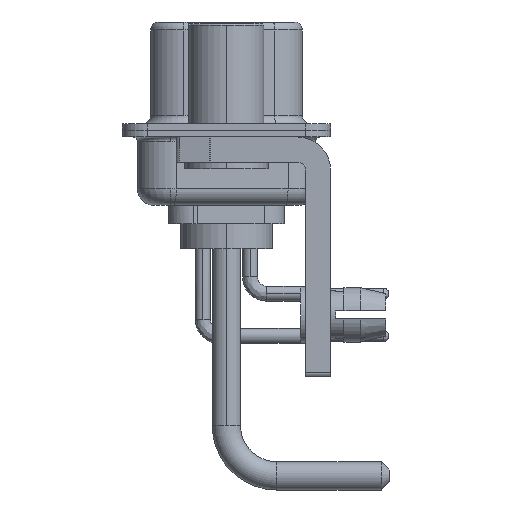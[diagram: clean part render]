
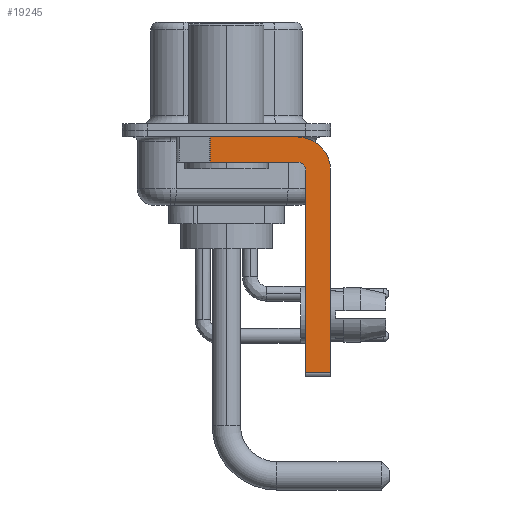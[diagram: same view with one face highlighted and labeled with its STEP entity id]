
A CAD part, left-side view. The second image highlights one B-rep face of the part: STEP entity #19245.
In plain terms, the highlighted planar face has unit normal (-1, 0, 0).
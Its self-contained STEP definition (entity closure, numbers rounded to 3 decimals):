
#707 = EDGE_CURVE ( 'NONE', #15622, #6679, #5319, .T. ) ;
#946 = CARTESIAN_POINT ( 'NONE',  ( -2.9, -4.75, -14.8 ) ) ;
#1296 = EDGE_CURVE ( 'NONE', #25440, #26084, #15263, .T. ) ;
#2064 = LINE ( 'NONE', #4436, #20215 ) ;
#2780 = VERTEX_POINT ( 'NONE', #26372 ) ;
#3285 = PLANE ( 'NONE',  #5467 ) ;
#3473 = DIRECTION ( 'NONE',  ( 0., 0., -1. ) ) ;
#4436 = CARTESIAN_POINT ( 'NONE',  ( -2.9, 3., -0.4 ) ) ;
#4575 = DIRECTION ( 'NONE',  ( 0., -1., 0. ) ) ;
#4729 = EDGE_CURVE ( 'NONE', #21478, #20223, #9816, .T. ) ;
#5319 = LINE ( 'NONE', #7099, #14915 ) ;
#5467 = AXIS2_PLACEMENT_3D ( 'NONE', #16999, #21433, #21286 ) ;
#5736 = ORIENTED_EDGE ( 'NONE', *, *, #15681, .F. ) ;
#5931 = DIRECTION ( 'NONE',  ( 0., 1., 0. ) ) ;
#6679 = VERTEX_POINT ( 'NONE', #17961 ) ;
#7099 = CARTESIAN_POINT ( 'NONE',  ( -2.9, 0.978, -1.9 ) ) ;
#7449 = DIRECTION ( 'NONE',  ( 0., 0., 1. ) ) ;
#7663 = CARTESIAN_POINT ( 'NONE',  ( -2.9, -4.25, -2.4 ) ) ;
#8130 = LINE ( 'NONE', #10212, #20425 ) ;
#9448 = DIRECTION ( 'NONE',  ( -1., 0., 0. ) ) ;
#9508 = CARTESIAN_POINT ( 'NONE',  ( -2.9, -4.25, -2.4 ) ) ;
#9785 = VECTOR ( 'NONE', #3473, 1000. ) ;
#9816 = LINE ( 'NONE', #946, #11301 ) ;
#9962 = VECTOR ( 'NONE', #14003, 1000. ) ;
#10212 = CARTESIAN_POINT ( 'NONE',  ( -2.9, -4.25, -1.9 ) ) ;
#11301 = VECTOR ( 'NONE', #7449, 1000. ) ;
#11596 = CARTESIAN_POINT ( 'NONE',  ( -2.9, -6.25, -2.4 ) ) ;
#11713 = EDGE_CURVE ( 'NONE', #21478, #26084, #15914, .T. ) ;
#12149 = FACE_OUTER_BOUND ( 'NONE', #17409, .T. ) ;
#13572 = CARTESIAN_POINT ( 'NONE',  ( -2.9, -4.25, -14.55 ) ) ;
#13869 = DIRECTION ( 'NONE',  ( 0., 0., 1. ) ) ;
#13924 = DIRECTION ( 'NONE',  ( 1., 0., 0. ) ) ;
#14003 = DIRECTION ( 'NONE',  ( 0., -1., 0. ) ) ;
#14226 = EDGE_CURVE ( 'NONE', #15622, #17719, #2064, .T. ) ;
#14915 = VECTOR ( 'NONE', #25531, 1000. ) ;
#15263 = LINE ( 'NONE', #21460, #9785 ) ;
#15462 = EDGE_CURVE ( 'NONE', #2780, #6679, #8130, .T. ) ;
#15622 = VERTEX_POINT ( 'NONE', #15921 ) ;
#15681 = EDGE_CURVE ( 'NONE', #20223, #2780, #28939, .T. ) ;
#15913 = ORIENTED_EDGE ( 'NONE', *, *, #14226, .F. ) ;
#15914 = LINE ( 'NONE', #13572, #9962 ) ;
#15921 = CARTESIAN_POINT ( 'NONE',  ( -2.9, 0.978, -0.4 ) ) ;
#16760 = ORIENTED_EDGE ( 'NONE', *, *, #11713, .T. ) ;
#16999 = CARTESIAN_POINT ( 'NONE',  ( -2.9, -4.25, -2.4 ) ) ;
#17387 = CARTESIAN_POINT ( 'NONE',  ( -2.9, -6.25, -14.55 ) ) ;
#17409 = EDGE_LOOP ( 'NONE', ( #15913, #19460, #28107, #5736, #18632, #16760, #27746, #24098 ) ) ;
#17719 = VERTEX_POINT ( 'NONE', #27190 ) ;
#17961 = CARTESIAN_POINT ( 'NONE',  ( -2.9, 0.978, -1.9 ) ) ;
#18492 = DIRECTION ( 'NONE',  ( 0., 0., -1. ) ) ;
#18632 = ORIENTED_EDGE ( 'NONE', *, *, #4729, .F. ) ;
#19245 = ADVANCED_FACE ( 'NONE', ( #12149 ), #3285, .F. ) ;
#19460 = ORIENTED_EDGE ( 'NONE', *, *, #707, .T. ) ;
#20215 = VECTOR ( 'NONE', #4575, 1000. ) ;
#20223 = VERTEX_POINT ( 'NONE', #28362 ) ;
#20425 = VECTOR ( 'NONE', #5931, 1000. ) ;
#21286 = DIRECTION ( 'NONE',  ( 0., 0., -1. ) ) ;
#21433 = DIRECTION ( 'NONE',  ( 1., 0., 0. ) ) ;
#21460 = CARTESIAN_POINT ( 'NONE',  ( -2.9, -6.25, -2.4 ) ) ;
#21478 = VERTEX_POINT ( 'NONE', #22788 ) ;
#22788 = CARTESIAN_POINT ( 'NONE',  ( -2.9, -4.75, -14.55 ) ) ;
#24098 = ORIENTED_EDGE ( 'NONE', *, *, #24456, .F. ) ;
#24456 = EDGE_CURVE ( 'NONE', #17719, #25440, #27776, .T. ) ;
#25440 = VERTEX_POINT ( 'NONE', #11596 ) ;
#25531 = DIRECTION ( 'NONE',  ( 0., 0., -1. ) ) ;
#26084 = VERTEX_POINT ( 'NONE', #17387 ) ;
#26372 = CARTESIAN_POINT ( 'NONE',  ( -2.9, -4.25, -1.9 ) ) ;
#27190 = CARTESIAN_POINT ( 'NONE',  ( -2.9, -4.25, -0.4 ) ) ;
#27541 = AXIS2_PLACEMENT_3D ( 'NONE', #7663, #9448, #13869 ) ;
#27746 = ORIENTED_EDGE ( 'NONE', *, *, #1296, .F. ) ;
#27776 = CIRCLE ( 'NONE', #28725, 2. ) ;
#28107 = ORIENTED_EDGE ( 'NONE', *, *, #15462, .F. ) ;
#28362 = CARTESIAN_POINT ( 'NONE',  ( -2.9, -4.75, -2.4 ) ) ;
#28725 = AXIS2_PLACEMENT_3D ( 'NONE', #9508, #13924, #18492 ) ;
#28939 = CIRCLE ( 'NONE', #27541, 0.5 ) ;
